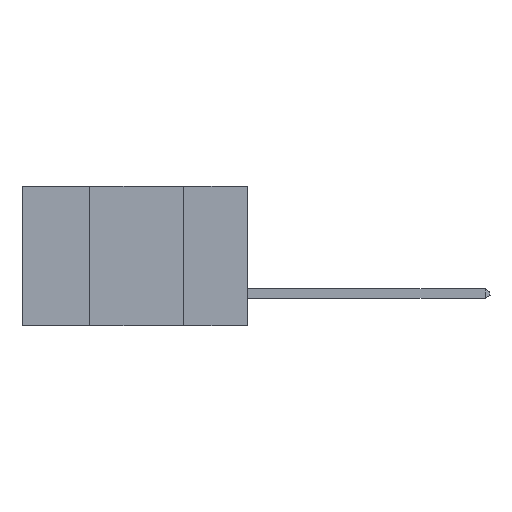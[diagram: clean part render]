
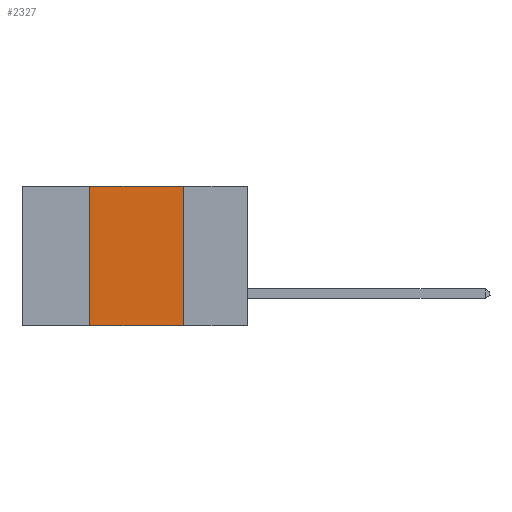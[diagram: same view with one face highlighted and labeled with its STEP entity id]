
A CAD part, left-side view. The second image highlights one B-rep face of the part: STEP entity #2327.
In plain terms, the highlighted planar face has unit normal (-1, 0, 0).
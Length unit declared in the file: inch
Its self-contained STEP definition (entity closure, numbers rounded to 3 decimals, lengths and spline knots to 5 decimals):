
#299 = ORIENTED_EDGE ( 'NONE', *, *, #7245, .F. ) ;
#1134 = CARTESIAN_POINT ( 'NONE',  ( 0., 0.17, -0.37 ) ) ;
#1713 = DIRECTION ( 'NONE',  ( 0., -1., 0. ) ) ;
#2035 = CARTESIAN_POINT ( 'NONE',  ( 0., 0.6, 0. ) ) ;
#2072 = VERTEX_POINT ( 'NONE', #3719 ) ;
#2233 = EDGE_CURVE ( 'NONE', #2072, #2726, #9796, .T. ) ;
#2327 = ADVANCED_FACE ( 'NONE', ( #8748 ), #3756, .F. ) ;
#2726 = VERTEX_POINT ( 'NONE', #4350 ) ;
#3029 = EDGE_CURVE ( 'NONE', #2072, #8966, #4381, .T. ) ;
#3096 = CARTESIAN_POINT ( 'NONE',  ( 0., 0.6, 0. ) ) ;
#3148 = CARTESIAN_POINT ( 'NONE',  ( 0., 0.6, -0.37 ) ) ;
#3170 = ORIENTED_EDGE ( 'NONE', *, *, #3244, .F. ) ;
#3244 = EDGE_CURVE ( 'NONE', #6665, #8966, #9101, .T. ) ;
#3427 = ORIENTED_EDGE ( 'NONE', *, *, #3029, .T. ) ;
#3544 = DIRECTION ( 'NONE',  ( 0., 0., -1. ) ) ;
#3601 = EDGE_LOOP ( 'NONE', ( #3170, #299, #6816, #3427 ) ) ;
#3719 = CARTESIAN_POINT ( 'NONE',  ( 0., 0.42, -0.37 ) ) ;
#3756 = PLANE ( 'NONE',  #8485 ) ;
#3909 = DIRECTION ( 'NONE',  ( 0., 0., -1. ) ) ;
#4350 = CARTESIAN_POINT ( 'NONE',  ( 0., 0.42, 0. ) ) ;
#4381 = LINE ( 'NONE', #3148, #4630 ) ;
#4531 = CARTESIAN_POINT ( 'NONE',  ( 0., 0.42, 0. ) ) ;
#4630 = VECTOR ( 'NONE', #1713, 39.37008 ) ;
#4878 = CARTESIAN_POINT ( 'NONE',  ( 0., 0.17, 0. ) ) ;
#5286 = DIRECTION ( 'NONE',  ( 0., 0., 1. ) ) ;
#6231 = LINE ( 'NONE', #2035, #6727 ) ;
#6665 = VERTEX_POINT ( 'NONE', #4878 ) ;
#6727 = VECTOR ( 'NONE', #6733, 39.37008 ) ;
#6733 = DIRECTION ( 'NONE',  ( 0., -1., 0. ) ) ;
#6816 = ORIENTED_EDGE ( 'NONE', *, *, #2233, .F. ) ;
#6951 = DIRECTION ( 'NONE',  ( 1., 0., 0. ) ) ;
#7066 = VECTOR ( 'NONE', #3544, 39.37008 ) ;
#7245 = EDGE_CURVE ( 'NONE', #2726, #6665, #6231, .T. ) ;
#8485 = AXIS2_PLACEMENT_3D ( 'NONE', #3096, #6951, #3909 ) ;
#8748 = FACE_OUTER_BOUND ( 'NONE', #3601, .T. ) ;
#8914 = CARTESIAN_POINT ( 'NONE',  ( 0., 0.17, 0. ) ) ;
#8966 = VERTEX_POINT ( 'NONE', #1134 ) ;
#9101 = LINE ( 'NONE', #8914, #7066 ) ;
#9546 = VECTOR ( 'NONE', #5286, 39.37008 ) ;
#9796 = LINE ( 'NONE', #4531, #9546 ) ;
